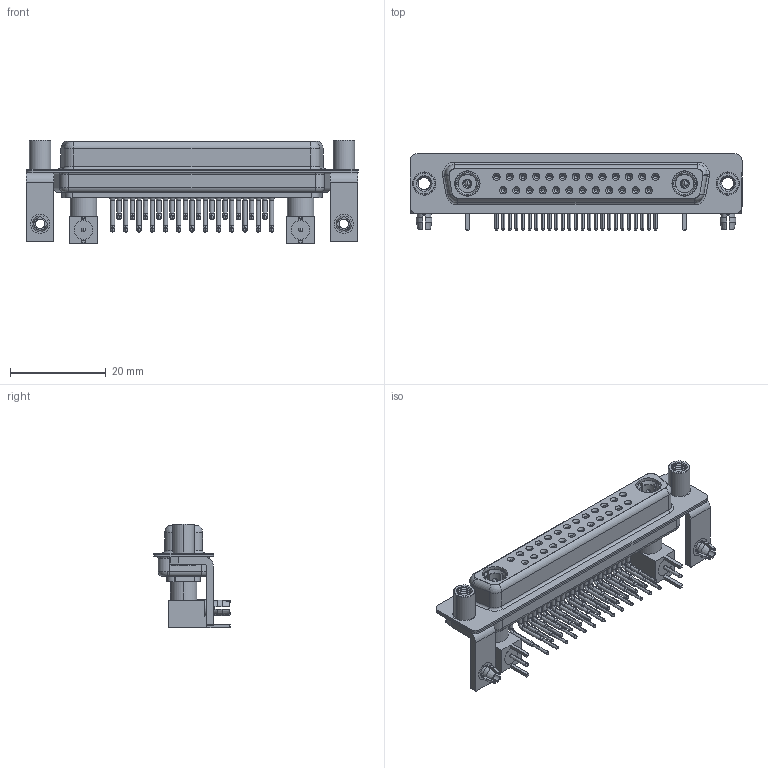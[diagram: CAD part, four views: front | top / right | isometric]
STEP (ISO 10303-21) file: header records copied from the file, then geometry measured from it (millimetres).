
FILE_DESCRIPTION (( 'STEP AP203' ), '1' );
FILE_NAME ('630-27W2240-5ND.STEP', '2022-06-07T13:00:15', ( '' ), ( '' ), 'SwSTEP 2.0', 'SolidWorks 2020', '' );
FILE_SCHEMA (( 'CONFIG_CONTROL_DESIGN' ));
Length unit declared in the file: millimetre
Products named in the file (17): Co-Ax Plug Assy_RA; 630Combo Shell Front_37 Contacts; 630Combo Threaded Standoff_D; 630Combo Contact Row 2; 630-27W2240-5ND; 630Combo Shell Rear_37 Contacts; 630Combo Stabilizer Bracket; 630Combo Housing_27W2; 630Combo Board Lock; Co-Ax Plug_RA PC Tail; Insulator RA Pin; Locking Collar; 630Combo Contact Row 1; RA Back Shell; Insulator Pin_Straight PC Tail; Pin_RA
Assembly tree (48 placements, depth 3):
  630-27W2240-5ND
    630Combo Housing_27W2
    630Combo Shell Front_37 Contacts
    630Combo Shell Rear_37 Contacts
    630Combo Stabilizer Bracket  x2
    630Combo Board Lock  x2
    630Combo Threaded Standoff_D  x2
    Co-Ax Plug Assy_RA
      Co-Ax Plug_RA PC Tail
      Insulator Pin_Straight PC Tail
      Pin_RA
      Locking Collar
      RA Back Shell
      Insulator RA Pin
    Co-Ax Plug Assy_RA
      Co-Ax Plug_RA PC Tail
      Insulator Pin_Straight PC Tail
      Pin_RA
      Locking Collar
      RA Back Shell
      Insulator RA Pin
    630Combo Contact Row 1  x13
    630Combo Contact Row 2  x12
Bounding box: 69.4 x 16 x 21.61 mm (x, y, z)
Volume: 6426.1 mm3; surface area: 14929.1 mm2
Topology: 46 solids, 46 shells, 2130 faces, 5376 edges, 3392 vertices
Faces by surface type: cylinder 946, plane 646, cone 353, bspline 108, torus 69, sphere 8
Entity records: 32222 total; most frequent: CARTESIAN_POINT 7498, DIRECTION 5020, ORIENTED_EDGE 4336, EDGE_CURVE 2168, AXIS2_PLACEMENT_3D 2062, VERTEX_POINT 1385, EDGE_LOOP 1109, CIRCLE 1102
